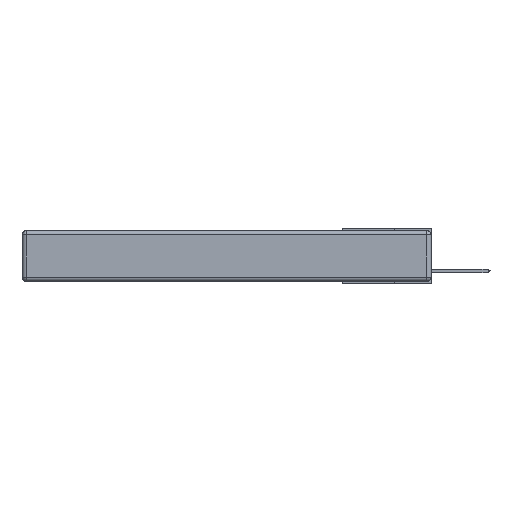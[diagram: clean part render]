
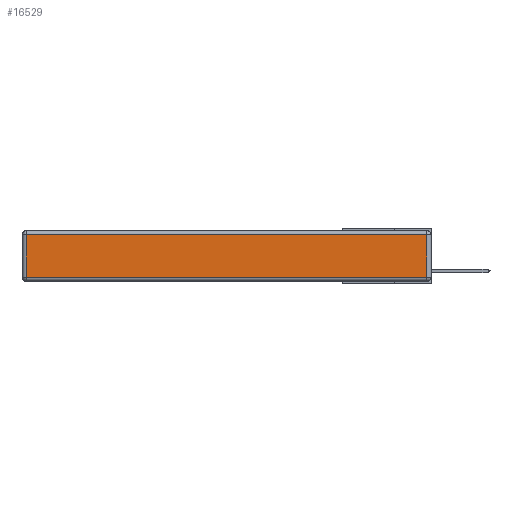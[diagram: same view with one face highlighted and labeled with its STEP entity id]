
A CAD part, left-side view. The second image highlights one B-rep face of the part: STEP entity #16529.
In plain terms, the highlighted planar face has unit normal (-1, 0, 0).
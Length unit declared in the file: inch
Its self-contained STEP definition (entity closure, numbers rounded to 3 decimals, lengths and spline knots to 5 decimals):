
#81 = DIRECTION ( 'NONE',  ( 0., 1., 0. ) ) ;
#226 = LINE ( 'NONE', #15149, #3277 ) ;
#612 = VERTEX_POINT ( 'NONE', #23970 ) ;
#1384 = DIRECTION ( 'NONE',  ( 0., -1., 0. ) ) ;
#2337 = DIRECTION ( 'NONE',  ( 0., 0., -1. ) ) ;
#3277 = VECTOR ( 'NONE', #81, 39.37008 ) ;
#5036 = ORIENTED_EDGE ( 'NONE', *, *, #22417, .T. ) ;
#5347 = EDGE_CURVE ( 'NONE', #16015, #18509, #6936, .T. ) ;
#5626 = VECTOR ( 'NONE', #2337, 39.37008 ) ;
#6163 = DIRECTION ( 'NONE',  ( 0., 0., 1. ) ) ;
#6452 = PLANE ( 'NONE',  #9975 ) ;
#6936 = LINE ( 'NONE', #10283, #9353 ) ;
#7087 = ORIENTED_EDGE ( 'NONE', *, *, #5347, .T. ) ;
#7884 = DIRECTION ( 'NONE',  ( 0., 0., 1. ) ) ;
#9021 = CARTESIAN_POINT ( 'NONE',  ( 0., 2.72, -0.313 ) ) ;
#9353 = VECTOR ( 'NONE', #7884, 39.37008 ) ;
#9975 = AXIS2_PLACEMENT_3D ( 'NONE', #17545, #17152, #6163 ) ;
#10131 = LINE ( 'NONE', #14739, #17724 ) ;
#10283 = CARTESIAN_POINT ( 'NONE',  ( 0., 0.03, -0.343 ) ) ;
#12743 = EDGE_LOOP ( 'NONE', ( #25463, #7087, #16601, #5036 ) ) ;
#12827 = LINE ( 'NONE', #13324, #5626 ) ;
#13324 = CARTESIAN_POINT ( 'NONE',  ( 0., 2.72, -0.343 ) ) ;
#14739 = CARTESIAN_POINT ( 'NONE',  ( 0., 0., -0.313 ) ) ;
#15149 = CARTESIAN_POINT ( 'NONE',  ( 0., 2.75, -0.03 ) ) ;
#15919 = EDGE_CURVE ( 'NONE', #18509, #612, #226, .T. ) ;
#16015 = VERTEX_POINT ( 'NONE', #24761 ) ;
#16529 = ADVANCED_FACE ( 'NONE', ( #17018 ), #6452, .T. ) ;
#16601 = ORIENTED_EDGE ( 'NONE', *, *, #15919, .T. ) ;
#17018 = FACE_OUTER_BOUND ( 'NONE', #12743, .T. ) ;
#17152 = DIRECTION ( 'NONE',  ( -1., 0., 0. ) ) ;
#17545 = CARTESIAN_POINT ( 'NONE',  ( 0., 0., -0.343 ) ) ;
#17724 = VECTOR ( 'NONE', #1384, 39.37008 ) ;
#18509 = VERTEX_POINT ( 'NONE', #19016 ) ;
#19016 = CARTESIAN_POINT ( 'NONE',  ( 0., 0.03, -0.03 ) ) ;
#20634 = VERTEX_POINT ( 'NONE', #9021 ) ;
#22082 = EDGE_CURVE ( 'NONE', #20634, #16015, #10131, .T. ) ;
#22417 = EDGE_CURVE ( 'NONE', #612, #20634, #12827, .T. ) ;
#23970 = CARTESIAN_POINT ( 'NONE',  ( 0., 2.72, -0.03 ) ) ;
#24761 = CARTESIAN_POINT ( 'NONE',  ( 0., 0.03, -0.313 ) ) ;
#25463 = ORIENTED_EDGE ( 'NONE', *, *, #22082, .T. ) ;
